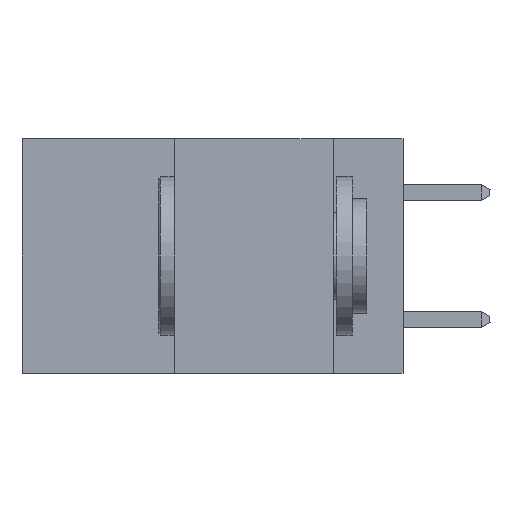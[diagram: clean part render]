
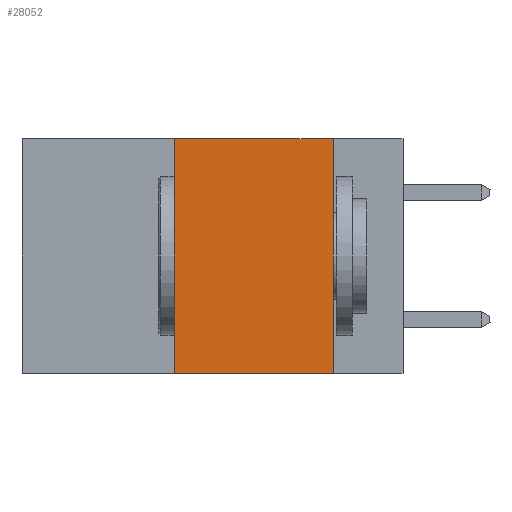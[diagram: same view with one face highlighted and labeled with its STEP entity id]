
A CAD part, left-side view. The second image highlights one B-rep face of the part: STEP entity #28052.
In plain terms, the highlighted planar face has unit normal (-1, 0, 0).
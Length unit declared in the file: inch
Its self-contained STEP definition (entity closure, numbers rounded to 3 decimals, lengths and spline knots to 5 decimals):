
#3741 = AXIS2_PLACEMENT_3D ( 'NONE', #21737, #40582, #47708 ) ;
#5980 = DIRECTION ( 'NONE',  ( 0., -1., 0. ) ) ;
#6887 = ORIENTED_EDGE ( 'NONE', *, *, #37535, .F. ) ;
#6967 = LINE ( 'NONE', #16170, #31895 ) ;
#8323 = CARTESIAN_POINT ( 'NONE',  ( 0., 0.11, 0. ) ) ;
#10047 = CARTESIAN_POINT ( 'NONE',  ( 0., 0.11, 0. ) ) ;
#12745 = DIRECTION ( 'NONE',  ( 0., 0., 1. ) ) ;
#13449 = EDGE_CURVE ( 'NONE', #14372, #24427, #37361, .T. ) ;
#14372 = VERTEX_POINT ( 'NONE', #8323 ) ;
#15194 = CARTESIAN_POINT ( 'NONE',  ( 0., 0.11, -0.37 ) ) ;
#15197 = VERTEX_POINT ( 'NONE', #24583 ) ;
#15743 = ORIENTED_EDGE ( 'NONE', *, *, #13449, .F. ) ;
#16170 = CARTESIAN_POINT ( 'NONE',  ( 0., 0.36, 0. ) ) ;
#17448 = LINE ( 'NONE', #32893, #42414 ) ;
#19160 = ORIENTED_EDGE ( 'NONE', *, *, #24131, .F. ) ;
#21737 = CARTESIAN_POINT ( 'NONE',  ( 0., 0.6, 0. ) ) ;
#23933 = VECTOR ( 'NONE', #44306, 39.37008 ) ;
#24131 = EDGE_CURVE ( 'NONE', #40189, #14372, #33098, .T. ) ;
#24341 = VECTOR ( 'NONE', #5980, 39.37008 ) ;
#24427 = VERTEX_POINT ( 'NONE', #15194 ) ;
#24583 = CARTESIAN_POINT ( 'NONE',  ( 0., 0.36, -0.37 ) ) ;
#25036 = CARTESIAN_POINT ( 'NONE',  ( 0., 0.6, 0. ) ) ;
#28052 = ADVANCED_FACE ( 'NONE', ( #29726 ), #36528, .F. ) ;
#28796 = EDGE_LOOP ( 'NONE', ( #15743, #19160, #6887, #46481 ) ) ;
#28983 = DIRECTION ( 'NONE',  ( 0., -1., 0. ) ) ;
#29726 = FACE_OUTER_BOUND ( 'NONE', #28796, .T. ) ;
#31895 = VECTOR ( 'NONE', #12745, 39.37008 ) ;
#32222 = CARTESIAN_POINT ( 'NONE',  ( 0., 0.36, 0. ) ) ;
#32893 = CARTESIAN_POINT ( 'NONE',  ( 0., 0.6, -0.37 ) ) ;
#33098 = LINE ( 'NONE', #25036, #24341 ) ;
#36528 = PLANE ( 'NONE',  #3741 ) ;
#37103 = EDGE_CURVE ( 'NONE', #15197, #24427, #17448, .T. ) ;
#37361 = LINE ( 'NONE', #10047, #23933 ) ;
#37535 = EDGE_CURVE ( 'NONE', #15197, #40189, #6967, .T. ) ;
#40189 = VERTEX_POINT ( 'NONE', #32222 ) ;
#40582 = DIRECTION ( 'NONE',  ( 1., 0., 0. ) ) ;
#42414 = VECTOR ( 'NONE', #28983, 39.37008 ) ;
#44306 = DIRECTION ( 'NONE',  ( 0., 0., -1. ) ) ;
#46481 = ORIENTED_EDGE ( 'NONE', *, *, #37103, .T. ) ;
#47708 = DIRECTION ( 'NONE',  ( 0., 0., -1. ) ) ;
